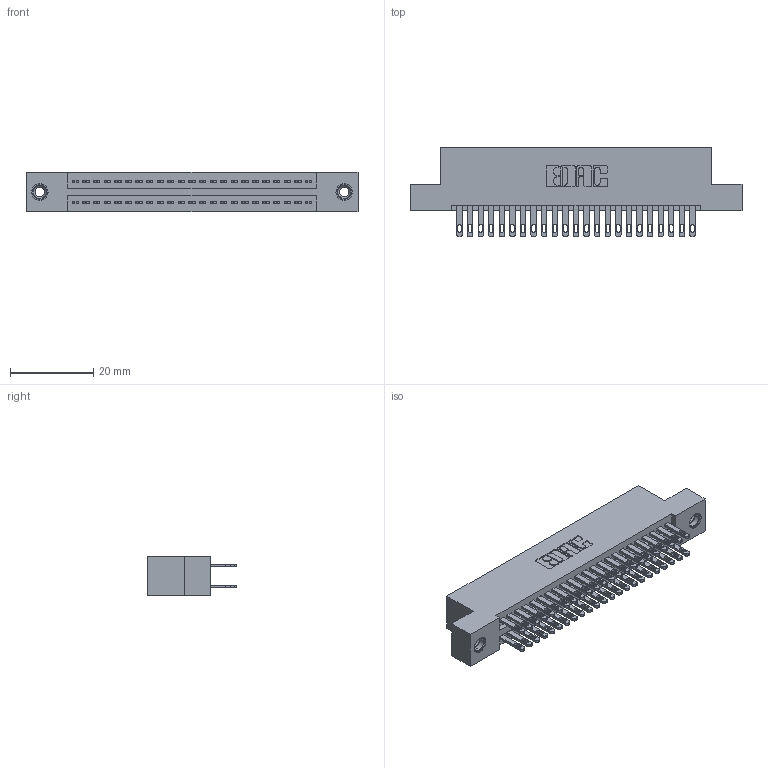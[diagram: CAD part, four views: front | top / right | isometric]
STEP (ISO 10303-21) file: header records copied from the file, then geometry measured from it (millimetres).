
FILE_DESCRIPTION (( 'STEP AP203' ), '1' );
FILE_NAME ('895-046-500-208.STEP', '2020-09-27T04:44:18', ( '' ), ( '' ), 'SwSTEP 2.0', 'SolidWorks 2020', '' );
FILE_SCHEMA (( 'CONFIG_CONTROL_DESIGN' ));
Length unit declared in the file: inch
Products named in the file (4): 345-250-001_345-250-003-102; 345-292-001_345-293-100; 845 Part_Flush Mounting Lugs - 0.156 Dia-TI; 895-046-500-208
Assembly tree (49 placements, depth 2):
  895-046-500-208
    845 Part_Flush Mounting Lugs - 0.156 Dia-TI
    345-292-001_345-293-100  x46
    345-250-001_345-250-003-102  x2
Bounding box: 79.63 x 21.51 x 9.4 mm (x, y, z)
Volume: 7692.9 mm3; surface area: 11486.1 mm2
Topology: 49 solids, 49 shells, 2302 faces, 6963 edges, 4634 vertices
Faces by surface type: plane 1354, cylinder 932, cone 12, torus 4
Entity records: 21720 total; most frequent: CARTESIAN_POINT 3639, ORIENTED_EDGE 3566, DIRECTION 3261, EDGE_CURVE 1783, LINE 1535, VECTOR 1535, VERTEX_POINT 1184, AXIS2_PLACEMENT_3D 863
